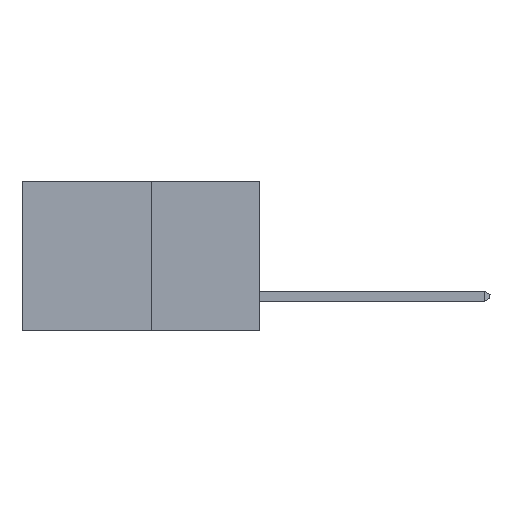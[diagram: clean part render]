
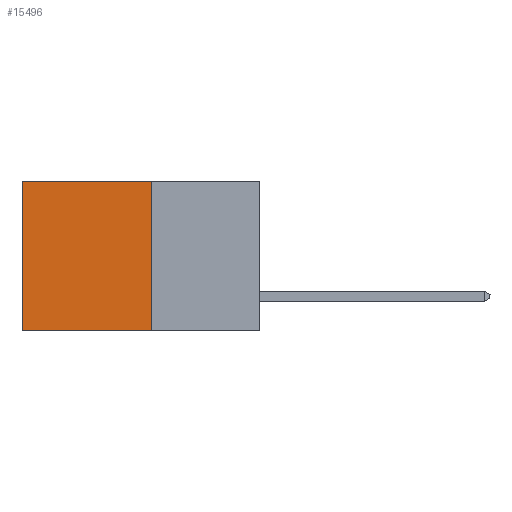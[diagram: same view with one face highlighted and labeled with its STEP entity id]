
A CAD part, left-side view. The second image highlights one B-rep face of the part: STEP entity #15496.
In plain terms, the highlighted planar face has unit normal (-1, 0, 0).
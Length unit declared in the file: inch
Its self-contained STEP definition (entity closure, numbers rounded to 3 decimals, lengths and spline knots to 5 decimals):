
#338 = DIRECTION ( 'NONE',  ( 0., 0., -1. ) ) ;
#551 = LINE ( 'NONE', #14963, #14584 ) ;
#1633 = CARTESIAN_POINT ( 'NONE',  ( 0.277, 0.27, -0.37 ) ) ;
#2477 = FACE_OUTER_BOUND ( 'NONE', #9804, .T. ) ;
#3814 = VECTOR ( 'NONE', #5396, 39.37008 ) ;
#3890 = VERTEX_POINT ( 'NONE', #12454 ) ;
#3912 = CARTESIAN_POINT ( 'NONE',  ( 0.277, 0.27, -0.37 ) ) ;
#4045 = ORIENTED_EDGE ( 'NONE', *, *, #13162, .F. ) ;
#4138 = EDGE_CURVE ( 'NONE', #14109, #7673, #551, .T. ) ;
#5396 = DIRECTION ( 'NONE',  ( 0., 0., -1. ) ) ;
#5884 = DIRECTION ( 'NONE',  ( 0., 0., -1. ) ) ;
#6276 = LINE ( 'NONE', #3912, #16435 ) ;
#6724 = CARTESIAN_POINT ( 'NONE',  ( 0.277, 0.59, -0.37 ) ) ;
#6980 = CARTESIAN_POINT ( 'NONE',  ( 0.277, 0.59, 0. ) ) ;
#7487 = LINE ( 'NONE', #6724, #3814 ) ;
#7673 = VERTEX_POINT ( 'NONE', #6980 ) ;
#7762 = ORIENTED_EDGE ( 'NONE', *, *, #15520, .F. ) ;
#8772 = CARTESIAN_POINT ( 'NONE',  ( 0.277, 0.27, -0.37 ) ) ;
#9387 = EDGE_CURVE ( 'NONE', #7673, #3890, #7487, .T. ) ;
#9513 = DIRECTION ( 'NONE',  ( 0., 1., 0. ) ) ;
#9804 = EDGE_LOOP ( 'NONE', ( #16722, #4045, #7762, #12408 ) ) ;
#10053 = PLANE ( 'NONE',  #14595 ) ;
#10433 = VERTEX_POINT ( 'NONE', #15376 ) ;
#12408 = ORIENTED_EDGE ( 'NONE', *, *, #4138, .T. ) ;
#12454 = CARTESIAN_POINT ( 'NONE',  ( 0.277, 0.59, -0.37 ) ) ;
#13162 = EDGE_CURVE ( 'NONE', #10433, #3890, #6276, .T. ) ;
#13322 = VECTOR ( 'NONE', #338, 39.37008 ) ;
#13881 = DIRECTION ( 'NONE',  ( 1., 0., 0. ) ) ;
#14109 = VERTEX_POINT ( 'NONE', #16157 ) ;
#14584 = VECTOR ( 'NONE', #17356, 39.37008 ) ;
#14595 = AXIS2_PLACEMENT_3D ( 'NONE', #1633, #13881, #5884 ) ;
#14963 = CARTESIAN_POINT ( 'NONE',  ( 0.277, 0.27, 0. ) ) ;
#15376 = CARTESIAN_POINT ( 'NONE',  ( 0.277, 0.27, -0.37 ) ) ;
#15496 = ADVANCED_FACE ( 'NONE', ( #2477 ), #10053, .F. ) ;
#15520 = EDGE_CURVE ( 'NONE', #14109, #10433, #15960, .T. ) ;
#15960 = LINE ( 'NONE', #8772, #13322 ) ;
#16157 = CARTESIAN_POINT ( 'NONE',  ( 0.277, 0.27, 0. ) ) ;
#16435 = VECTOR ( 'NONE', #9513, 39.37008 ) ;
#16722 = ORIENTED_EDGE ( 'NONE', *, *, #9387, .T. ) ;
#17356 = DIRECTION ( 'NONE',  ( 0., 1., 0. ) ) ;
